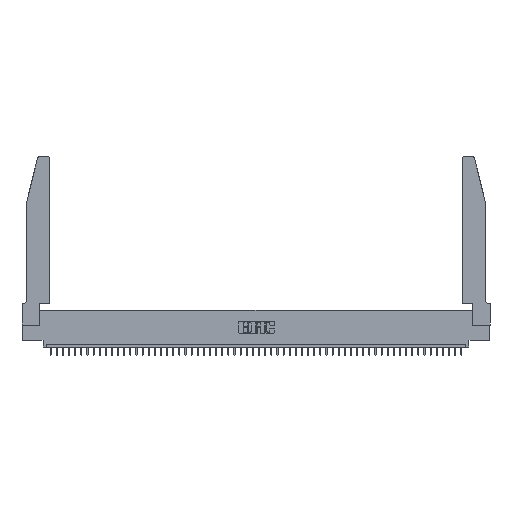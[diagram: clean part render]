
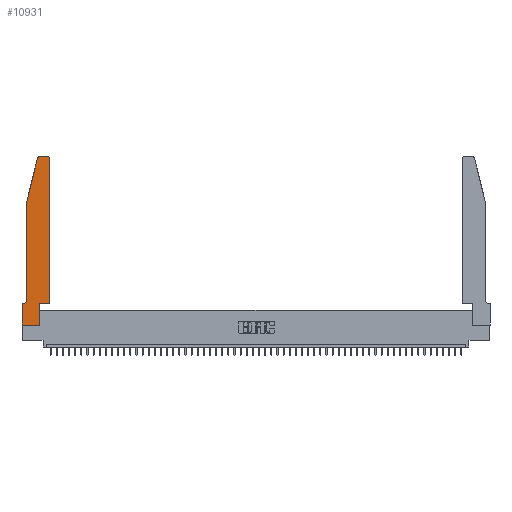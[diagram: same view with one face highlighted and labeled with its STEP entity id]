
A CAD part, top view. The second image highlights one B-rep face of the part: STEP entity #10931.
In plain terms, the highlighted planar face has unit normal (0, 0, 1).
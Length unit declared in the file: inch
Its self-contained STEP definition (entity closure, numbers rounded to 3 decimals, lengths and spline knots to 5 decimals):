
#1257 = CARTESIAN_POINT ( 'NONE',  ( 0.0055, 0.35, 0.37 ) ) ;
#1461 = DIRECTION ( 'NONE',  ( -1., 0., 0. ) ) ;
#1572 = PLANE ( 'NONE',  #25747 ) ;
#1927 = EDGE_CURVE ( 'NONE', #31543, #44904, #2726, .T. ) ;
#2090 = LINE ( 'NONE', #47109, #19179 ) ;
#2126 = CARTESIAN_POINT ( 'NONE',  ( 0.4505, 0.35, 0.37 ) ) ;
#2467 = AXIS2_PLACEMENT_3D ( 'NONE', #35393, #13676, #12887 ) ;
#2471 = DIRECTION ( 'NONE',  ( 1., 0., 0. ) ) ;
#2726 = LINE ( 'NONE', #10469, #13075 ) ;
#3966 = VERTEX_POINT ( 'NONE', #25315 ) ;
#4588 = VECTOR ( 'NONE', #35597, 39.37008 ) ;
#4618 = CARTESIAN_POINT ( 'NONE',  ( 0.4205, 2.72, 0.37 ) ) ;
#5111 = CIRCLE ( 'NONE', #22113, 0.03 ) ;
#5420 = DIRECTION ( 'NONE',  ( 1., 0., 0. ) ) ;
#5552 = CARTESIAN_POINT ( 'NONE',  ( 0.0755, 2., 0.37 ) ) ;
#6240 = DIRECTION ( 'NONE',  ( 0., -1., 0. ) ) ;
#6663 = LINE ( 'NONE', #2126, #51071 ) ;
#7023 = ORIENTED_EDGE ( 'NONE', *, *, #21143, .T. ) ;
#7247 = CARTESIAN_POINT ( 'NONE',  ( 0., 0., 0.37 ) ) ;
#7819 = LINE ( 'NONE', #24057, #23810 ) ;
#7984 = CARTESIAN_POINT ( 'NONE',  ( 0.4505, 0.35, 0.37 ) ) ;
#8495 = EDGE_CURVE ( 'NONE', #27472, #31543, #17231, .T. ) ;
#9158 = CARTESIAN_POINT ( 'NONE',  ( 0.284, 2.72, 0.37 ) ) ;
#9809 = ORIENTED_EDGE ( 'NONE', *, *, #24251, .T. ) ;
#10469 = CARTESIAN_POINT ( 'NONE',  ( 0., 0., 0.37 ) ) ;
#10931 = ADVANCED_FACE ( 'NONE', ( #37569 ), #1572, .T. ) ;
#11301 = ORIENTED_EDGE ( 'NONE', *, *, #49421, .T. ) ;
#11377 = VERTEX_POINT ( 'NONE', #1257 ) ;
#12035 = VERTEX_POINT ( 'NONE', #38590 ) ;
#12887 = DIRECTION ( 'NONE',  ( -1., 0., 0. ) ) ;
#13075 = VECTOR ( 'NONE', #2471, 39.37008 ) ;
#13615 = CARTESIAN_POINT ( 'NONE',  ( 0.4205, 2.75, 0.37 ) ) ;
#13676 = DIRECTION ( 'NONE',  ( 0., 0., -1. ) ) ;
#13755 = CARTESIAN_POINT ( 'NONE',  ( 0.284, 2.75, 0.37 ) ) ;
#13986 = EDGE_LOOP ( 'NONE', ( #44321, #7023, #21603, #9809, #41213, #38054, #27163, #27370, #50733, #46760, #43011, #11301 ) ) ;
#14169 = DIRECTION ( 'NONE',  ( 1., 0., 0. ) ) ;
#14998 = EDGE_CURVE ( 'NONE', #11377, #27472, #36394, .T. ) ;
#15295 = CARTESIAN_POINT ( 'NONE',  ( 0.4505, 2.72, 0.37 ) ) ;
#16652 = VERTEX_POINT ( 'NONE', #13615 ) ;
#16957 = CIRCLE ( 'NONE', #2467, 0.07 ) ;
#17169 = EDGE_CURVE ( 'NONE', #44904, #3966, #2090, .T. ) ;
#17231 = LINE ( 'NONE', #37752, #45252 ) ;
#17612 = VERTEX_POINT ( 'NONE', #13755 ) ;
#17837 = DIRECTION ( 'NONE',  ( 0., 0., 1. ) ) ;
#18350 = DIRECTION ( 'NONE',  ( 0., 1., 0. ) ) ;
#19179 = VECTOR ( 'NONE', #18350, 39.37008 ) ;
#20203 = EDGE_CURVE ( 'NONE', #44500, #12035, #30052, .T. ) ;
#20589 = DIRECTION ( 'NONE',  ( 1., 0., 0. ) ) ;
#20860 = DIRECTION ( 'NONE',  ( 0., 0., 1. ) ) ;
#21143 = EDGE_CURVE ( 'NONE', #17612, #44500, #32241, .T. ) ;
#21603 = ORIENTED_EDGE ( 'NONE', *, *, #20203, .T. ) ;
#22113 = AXIS2_PLACEMENT_3D ( 'NONE', #4618, #20860, #20589 ) ;
#22863 = VERTEX_POINT ( 'NONE', #7984 ) ;
#23290 = EDGE_CURVE ( 'NONE', #36936, #11377, #16957, .T. ) ;
#23810 = VECTOR ( 'NONE', #14169, 39.37008 ) ;
#24057 = CARTESIAN_POINT ( 'NONE',  ( 0.4505, 0.35, 0.37 ) ) ;
#24251 = EDGE_CURVE ( 'NONE', #12035, #36936, #42722, .T. ) ;
#25116 = CARTESIAN_POINT ( 'NONE',  ( 0.2865, 0., 0.37 ) ) ;
#25315 = CARTESIAN_POINT ( 'NONE',  ( 0.2865, 0.35, 0.37 ) ) ;
#25410 = DIRECTION ( 'NONE',  ( 0., 0., 1. ) ) ;
#25747 = AXIS2_PLACEMENT_3D ( 'NONE', #37309, #17837, #50308 ) ;
#25963 = CARTESIAN_POINT ( 'NONE',  ( 0.0755, 2., 0.37 ) ) ;
#26382 = VECTOR ( 'NONE', #6240, 39.37008 ) ;
#26533 = DIRECTION ( 'NONE',  ( 0., -1., 0. ) ) ;
#26641 = VERTEX_POINT ( 'NONE', #15295 ) ;
#26871 = CARTESIAN_POINT ( 'NONE',  ( 0.0755, 0.42, 0.37 ) ) ;
#27163 = ORIENTED_EDGE ( 'NONE', *, *, #8495, .T. ) ;
#27370 = ORIENTED_EDGE ( 'NONE', *, *, #1927, .T. ) ;
#27472 = VERTEX_POINT ( 'NONE', #31957 ) ;
#28226 = EDGE_CURVE ( 'NONE', #16652, #17612, #49683, .T. ) ;
#30052 = LINE ( 'NONE', #5552, #40686 ) ;
#31543 = VERTEX_POINT ( 'NONE', #7247 ) ;
#31957 = CARTESIAN_POINT ( 'NONE',  ( 0., 0.35, 0.37 ) ) ;
#32241 = CIRCLE ( 'NONE', #47549, 0.03 ) ;
#35393 = CARTESIAN_POINT ( 'NONE',  ( 0.0055, 0.42, 0.37 ) ) ;
#35597 = DIRECTION ( 'NONE',  ( -1., 0., 0. ) ) ;
#36394 = LINE ( 'NONE', #51808, #4588 ) ;
#36936 = VERTEX_POINT ( 'NONE', #26871 ) ;
#37309 = CARTESIAN_POINT ( 'NONE',  ( 0., 0.35, 0.37 ) ) ;
#37569 = FACE_OUTER_BOUND ( 'NONE', #13986, .T. ) ;
#37752 = CARTESIAN_POINT ( 'NONE',  ( 0., 0., 0.37 ) ) ;
#38054 = ORIENTED_EDGE ( 'NONE', *, *, #14998, .T. ) ;
#38590 = CARTESIAN_POINT ( 'NONE',  ( 0.0755, 2., 0.37 ) ) ;
#38640 = DIRECTION ( 'NONE',  ( 0., 1., 0. ) ) ;
#40686 = VECTOR ( 'NONE', #45235, 39.37008 ) ;
#41213 = ORIENTED_EDGE ( 'NONE', *, *, #23290, .T. ) ;
#42203 = CARTESIAN_POINT ( 'NONE',  ( 0.25487, 2.72718, 0.37 ) ) ;
#42722 = LINE ( 'NONE', #25963, #26382 ) ;
#43011 = ORIENTED_EDGE ( 'NONE', *, *, #51289, .T. ) ;
#44126 = VECTOR ( 'NONE', #1461, 39.37008 ) ;
#44321 = ORIENTED_EDGE ( 'NONE', *, *, #28226, .T. ) ;
#44500 = VERTEX_POINT ( 'NONE', #42203 ) ;
#44904 = VERTEX_POINT ( 'NONE', #25116 ) ;
#45235 = DIRECTION ( 'NONE',  ( -0.239, -0.971, 0. ) ) ;
#45252 = VECTOR ( 'NONE', #26533, 39.37008 ) ;
#46760 = ORIENTED_EDGE ( 'NONE', *, *, #49445, .T. ) ;
#47109 = CARTESIAN_POINT ( 'NONE',  ( 0.2865, 0.35, 0.37 ) ) ;
#47549 = AXIS2_PLACEMENT_3D ( 'NONE', #9158, #25410, #5420 ) ;
#49166 = CARTESIAN_POINT ( 'NONE',  ( 0.2605, 2.75, 0.37 ) ) ;
#49421 = EDGE_CURVE ( 'NONE', #26641, #16652, #5111, .T. ) ;
#49445 = EDGE_CURVE ( 'NONE', #3966, #22863, #7819, .T. ) ;
#49683 = LINE ( 'NONE', #49166, #44126 ) ;
#50308 = DIRECTION ( 'NONE',  ( 1., 0., 0. ) ) ;
#50733 = ORIENTED_EDGE ( 'NONE', *, *, #17169, .T. ) ;
#51071 = VECTOR ( 'NONE', #38640, 39.37008 ) ;
#51289 = EDGE_CURVE ( 'NONE', #22863, #26641, #6663, .T. ) ;
#51808 = CARTESIAN_POINT ( 'NONE',  ( 0.0755, 0.35, 0.37 ) ) ;
